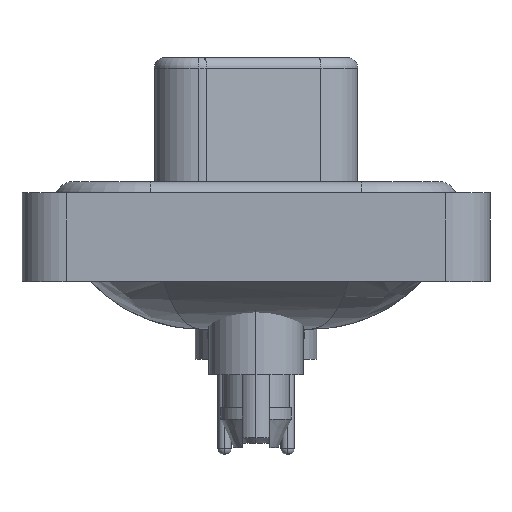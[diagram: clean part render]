
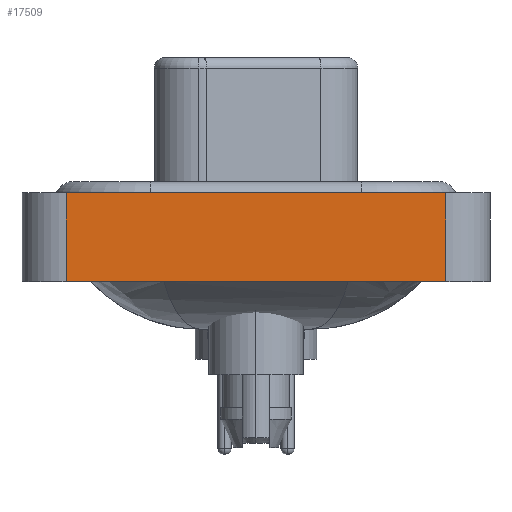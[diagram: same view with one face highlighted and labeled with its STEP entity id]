
A CAD part, left-side view. The second image highlights one B-rep face of the part: STEP entity #17509.
In plain terms, the highlighted planar face has unit normal (-1, 0, 0).
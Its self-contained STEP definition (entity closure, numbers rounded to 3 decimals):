
#133 = VERTEX_POINT ( 'NONE', #19815 ) ;
#248 = ORIENTED_EDGE ( 'NONE', *, *, #1079, .F. ) ;
#914 = LINE ( 'NONE', #10323, #16333 ) ;
#1079 = EDGE_CURVE ( 'NONE', #19769, #133, #3431, .T. ) ;
#2652 = ORIENTED_EDGE ( 'NONE', *, *, #24157, .F. ) ;
#3431 = LINE ( 'NONE', #24596, #15042 ) ;
#4232 = EDGE_CURVE ( 'NONE', #16305, #5102, #914, .T. ) ;
#4557 = FACE_OUTER_BOUND ( 'NONE', #17507, .T. ) ;
#4835 = CARTESIAN_POINT ( 'NONE',  ( -7.35, 8.55, -3.6 ) ) ;
#5102 = VERTEX_POINT ( 'NONE', #9600 ) ;
#5747 = EDGE_CURVE ( 'NONE', #5102, #133, #10535, .T. ) ;
#6583 = DIRECTION ( 'NONE',  ( -1., 0., 0. ) ) ;
#6593 = CARTESIAN_POINT ( 'NONE',  ( -7.35, -8.55, -3.6 ) ) ;
#8365 = DIRECTION ( 'NONE',  ( 0., 0., 1. ) ) ;
#8468 = ORIENTED_EDGE ( 'NONE', *, *, #5747, .T. ) ;
#8770 = DIRECTION ( 'NONE',  ( 0., 0., 1. ) ) ;
#8913 = DIRECTION ( 'NONE',  ( 0., -1., 0. ) ) ;
#9600 = CARTESIAN_POINT ( 'NONE',  ( -7.35, -8.55, -3.6 ) ) ;
#10323 = CARTESIAN_POINT ( 'NONE',  ( -7.35, -8.55, -3.6 ) ) ;
#10535 = LINE ( 'NONE', #6593, #13177 ) ;
#12280 = PLANE ( 'NONE',  #22945 ) ;
#12926 = DIRECTION ( 'NONE',  ( 0., -1., 0. ) ) ;
#13177 = VECTOR ( 'NONE', #8770, 1000. ) ;
#14311 = DIRECTION ( 'NONE',  ( 0., 0., 1. ) ) ;
#15042 = VECTOR ( 'NONE', #8913, 1000. ) ;
#15459 = CARTESIAN_POINT ( 'NONE',  ( -7.35, 8.55, 0.4 ) ) ;
#16211 = LINE ( 'NONE', #4835, #18291 ) ;
#16305 = VERTEX_POINT ( 'NONE', #16701 ) ;
#16333 = VECTOR ( 'NONE', #12926, 1000. ) ;
#16701 = CARTESIAN_POINT ( 'NONE',  ( -7.35, 8.55, -3.6 ) ) ;
#17507 = EDGE_LOOP ( 'NONE', ( #8468, #248, #2652, #22109 ) ) ;
#17509 = ADVANCED_FACE ( 'NONE', ( #4557 ), #12280, .T. ) ;
#18291 = VECTOR ( 'NONE', #8365, 1000. ) ;
#19769 = VERTEX_POINT ( 'NONE', #15459 ) ;
#19815 = CARTESIAN_POINT ( 'NONE',  ( -7.35, -8.55, 0.4 ) ) ;
#22109 = ORIENTED_EDGE ( 'NONE', *, *, #4232, .T. ) ;
#22945 = AXIS2_PLACEMENT_3D ( 'NONE', #23942, #6583, #14311 ) ;
#23942 = CARTESIAN_POINT ( 'NONE',  ( -7.35, -8.55, -3.6 ) ) ;
#24157 = EDGE_CURVE ( 'NONE', #16305, #19769, #16211, .T. ) ;
#24596 = CARTESIAN_POINT ( 'NONE',  ( -7.35, -8.55, 0.4 ) ) ;
